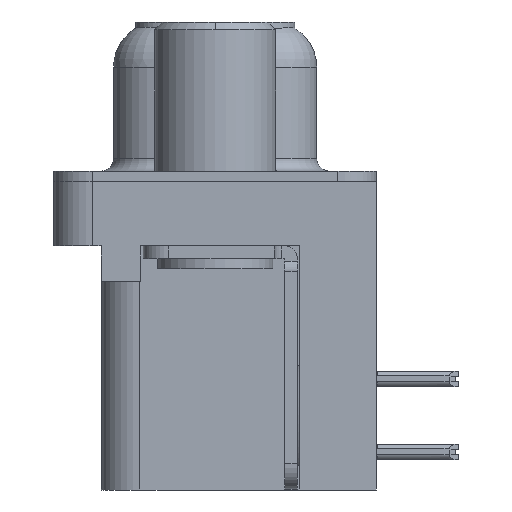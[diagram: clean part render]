
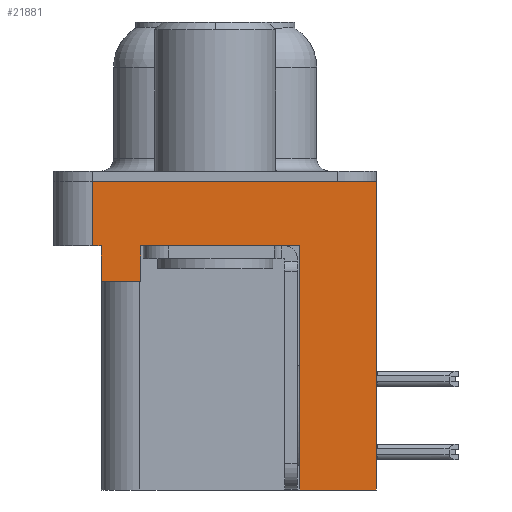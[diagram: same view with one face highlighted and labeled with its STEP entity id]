
A CAD part, left-side view. The second image highlights one B-rep face of the part: STEP entity #21881.
In plain terms, the highlighted planar face has unit normal (-1, 0, 0).
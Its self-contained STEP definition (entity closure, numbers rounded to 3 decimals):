
#894 = FACE_OUTER_BOUND ( 'NONE', #25643, .T. ) ;
#916 = LINE ( 'NONE', #19759, #16240 ) ;
#1117 = EDGE_CURVE ( 'NONE', #12715, #6625, #916, .T. ) ;
#1221 = VERTEX_POINT ( 'NONE', #13923 ) ;
#1501 = EDGE_CURVE ( 'NONE', #4645, #15318, #23404, .T. ) ;
#1786 = CARTESIAN_POINT ( 'NONE',  ( -2.91, -3.295, -12. ) ) ;
#1837 = ORIENTED_EDGE ( 'NONE', *, *, #1117, .F. ) ;
#1939 = DIRECTION ( 'NONE',  ( 0., 0., 1. ) ) ;
#1990 = CARTESIAN_POINT ( 'NONE',  ( -2.91, -6.275, -2.5 ) ) ;
#2009 = VECTOR ( 'NONE', #1939, 1000. ) ;
#2244 = CARTESIAN_POINT ( 'NONE',  ( -2.91, -6.275, 0. ) ) ;
#2469 = VERTEX_POINT ( 'NONE', #24088 ) ;
#2669 = LINE ( 'NONE', #1990, #22034 ) ;
#3193 = CARTESIAN_POINT ( 'NONE',  ( -2.91, 4.775, -2.5 ) ) ;
#3344 = ORIENTED_EDGE ( 'NONE', *, *, #1501, .F. ) ;
#3417 = CARTESIAN_POINT ( 'NONE',  ( -2.91, -3.295, -12. ) ) ;
#3703 = DIRECTION ( 'NONE',  ( 0., -1., 0. ) ) ;
#3874 = CARTESIAN_POINT ( 'NONE',  ( -2.91, -3.295, -12. ) ) ;
#4645 = VERTEX_POINT ( 'NONE', #9528 ) ;
#4732 = DIRECTION ( 'NONE',  ( 0., 1., 0. ) ) ;
#4918 = DIRECTION ( 'NONE',  ( -1., 0., 0. ) ) ;
#5132 = DIRECTION ( 'NONE',  ( 0., 0., 1. ) ) ;
#5522 = EDGE_CURVE ( 'NONE', #16228, #23234, #18566, .T. ) ;
#5825 = EDGE_CURVE ( 'NONE', #1221, #12715, #25012, .T. ) ;
#6381 = VERTEX_POINT ( 'NONE', #17431 ) ;
#6625 = VERTEX_POINT ( 'NONE', #2244 ) ;
#7011 = VECTOR ( 'NONE', #3703, 1000. ) ;
#7078 = EDGE_CURVE ( 'NONE', #15318, #6381, #19993, .T. ) ;
#7192 = PLANE ( 'NONE',  #8675 ) ;
#7219 = DIRECTION ( 'NONE',  ( 0., 0., 1. ) ) ;
#7619 = DIRECTION ( 'NONE',  ( 0., 1., 0. ) ) ;
#7886 = VECTOR ( 'NONE', #4732, 1000. ) ;
#8675 = AXIS2_PLACEMENT_3D ( 'NONE', #14970, #4918, #13062 ) ;
#8803 = ORIENTED_EDGE ( 'NONE', *, *, #16081, .T. ) ;
#9150 = CARTESIAN_POINT ( 'NONE',  ( -2.91, 2.895, -3.9 ) ) ;
#9528 = CARTESIAN_POINT ( 'NONE',  ( -2.91, -6.275, -12. ) ) ;
#9551 = LINE ( 'NONE', #10507, #12987 ) ;
#9701 = ORIENTED_EDGE ( 'NONE', *, *, #12014, .T. ) ;
#9824 = CARTESIAN_POINT ( 'NONE',  ( -2.91, 4.425, -3.9 ) ) ;
#10384 = VECTOR ( 'NONE', #7219, 1000. ) ;
#10507 = CARTESIAN_POINT ( 'NONE',  ( -2.91, -6.275, -2.5 ) ) ;
#11115 = ORIENTED_EDGE ( 'NONE', *, *, #7078, .F. ) ;
#11183 = LINE ( 'NONE', #9150, #24566 ) ;
#12014 = EDGE_CURVE ( 'NONE', #4645, #6625, #2669, .T. ) ;
#12633 = CARTESIAN_POINT ( 'NONE',  ( -2.91, 4.425, -3.9 ) ) ;
#12715 = VERTEX_POINT ( 'NONE', #16724 ) ;
#12987 = VECTOR ( 'NONE', #22176, 1000. ) ;
#13062 = DIRECTION ( 'NONE',  ( 0., 0., 1. ) ) ;
#13175 = ORIENTED_EDGE ( 'NONE', *, *, #14451, .F. ) ;
#13410 = VECTOR ( 'NONE', #7619, 1000. ) ;
#13923 = CARTESIAN_POINT ( 'NONE',  ( -2.91, 4.775, -2.5 ) ) ;
#14451 = EDGE_CURVE ( 'NONE', #24004, #16228, #22571, .T. ) ;
#14970 = CARTESIAN_POINT ( 'NONE',  ( -2.91, -6.275, -2.5 ) ) ;
#15318 = VERTEX_POINT ( 'NONE', #3874 ) ;
#15603 = CARTESIAN_POINT ( 'NONE',  ( -2.91, 4.425, -3.9 ) ) ;
#15760 = DIRECTION ( 'NONE',  ( 0., 0., 1. ) ) ;
#16081 = EDGE_CURVE ( 'NONE', #2469, #6381, #9551, .T. ) ;
#16228 = VERTEX_POINT ( 'NONE', #15603 ) ;
#16240 = VECTOR ( 'NONE', #19501, 1000. ) ;
#16724 = CARTESIAN_POINT ( 'NONE',  ( -2.91, 4.775, 0. ) ) ;
#17010 = CARTESIAN_POINT ( 'NONE',  ( -2.91, 4.425, -2.5 ) ) ;
#17431 = CARTESIAN_POINT ( 'NONE',  ( -2.91, -3.295, -2.5 ) ) ;
#17435 = EDGE_CURVE ( 'NONE', #1221, #23234, #21704, .T. ) ;
#17889 = DIRECTION ( 'NONE',  ( 0., 0., 1. ) ) ;
#17949 = CARTESIAN_POINT ( 'NONE',  ( -2.91, -6.275, -2.5 ) ) ;
#18566 = LINE ( 'NONE', #9824, #2009 ) ;
#18762 = ORIENTED_EDGE ( 'NONE', *, *, #23295, .T. ) ;
#19049 = VECTOR ( 'NONE', #15760, 1000. ) ;
#19254 = ORIENTED_EDGE ( 'NONE', *, *, #17435, .T. ) ;
#19501 = DIRECTION ( 'NONE',  ( 0., -1., 0. ) ) ;
#19759 = CARTESIAN_POINT ( 'NONE',  ( -2.91, -6.275, 0. ) ) ;
#19993 = LINE ( 'NONE', #1786, #19049 ) ;
#21007 = CARTESIAN_POINT ( 'NONE',  ( -2.91, 2.895, -3.9 ) ) ;
#21704 = LINE ( 'NONE', #17949, #7011 ) ;
#21881 = ADVANCED_FACE ( 'NONE', ( #894 ), #7192, .T. ) ;
#22034 = VECTOR ( 'NONE', #17889, 1000. ) ;
#22165 = ORIENTED_EDGE ( 'NONE', *, *, #5522, .F. ) ;
#22176 = DIRECTION ( 'NONE',  ( 0., -1., 0. ) ) ;
#22571 = LINE ( 'NONE', #12633, #7886 ) ;
#22976 = ORIENTED_EDGE ( 'NONE', *, *, #5825, .F. ) ;
#23234 = VERTEX_POINT ( 'NONE', #17010 ) ;
#23295 = EDGE_CURVE ( 'NONE', #24004, #2469, #11183, .T. ) ;
#23404 = LINE ( 'NONE', #3417, #13410 ) ;
#24004 = VERTEX_POINT ( 'NONE', #21007 ) ;
#24088 = CARTESIAN_POINT ( 'NONE',  ( -2.91, 2.895, -2.5 ) ) ;
#24566 = VECTOR ( 'NONE', #5132, 1000. ) ;
#25012 = LINE ( 'NONE', #3193, #10384 ) ;
#25643 = EDGE_LOOP ( 'NONE', ( #1837, #22976, #19254, #22165, #13175, #18762, #8803, #11115, #3344, #9701 ) ) ;
